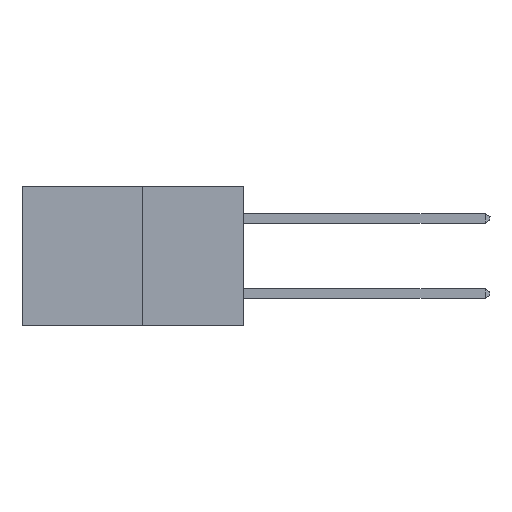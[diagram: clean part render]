
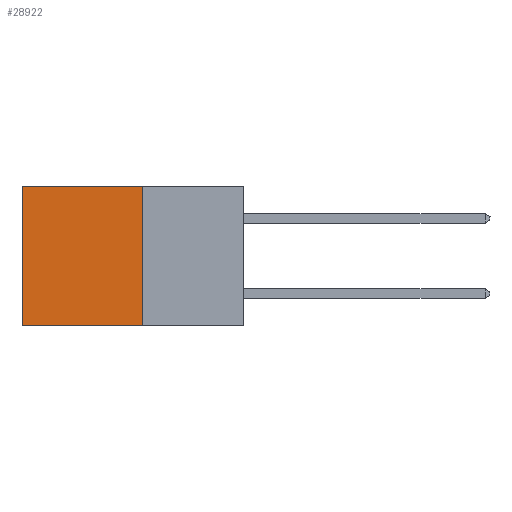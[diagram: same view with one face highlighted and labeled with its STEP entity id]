
A CAD part, left-side view. The second image highlights one B-rep face of the part: STEP entity #28922.
In plain terms, the highlighted planar face has unit normal (-1, 0, 0).
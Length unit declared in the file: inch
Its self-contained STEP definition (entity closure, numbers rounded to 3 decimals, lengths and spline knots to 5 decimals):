
#499 = CARTESIAN_POINT ( 'NONE',  ( 0.277, 0.59, 0. ) ) ;
#1030 = DIRECTION ( 'NONE',  ( 0., 0., -1. ) ) ;
#1636 = DIRECTION ( 'NONE',  ( 0., 0., -1. ) ) ;
#2954 = LINE ( 'NONE', #26502, #8799 ) ;
#3032 = LINE ( 'NONE', #10955, #22150 ) ;
#5028 = VECTOR ( 'NONE', #32125, 39.37008 ) ;
#6958 = PLANE ( 'NONE',  #21316 ) ;
#8799 = VECTOR ( 'NONE', #9034, 39.37008 ) ;
#9034 = DIRECTION ( 'NONE',  ( 0., 1., 0. ) ) ;
#10135 = ORIENTED_EDGE ( 'NONE', *, *, #14363, .F. ) ;
#10955 = CARTESIAN_POINT ( 'NONE',  ( 0.277, 0.27, -0.37 ) ) ;
#11963 = CARTESIAN_POINT ( 'NONE',  ( 0.277, 0.27, -0.37 ) ) ;
#12255 = ORIENTED_EDGE ( 'NONE', *, *, #31944, .T. ) ;
#13295 = FACE_OUTER_BOUND ( 'NONE', #19484, .T. ) ;
#14037 = EDGE_CURVE ( 'NONE', #16642, #22897, #18237, .T. ) ;
#14363 = EDGE_CURVE ( 'NONE', #31756, #16642, #3032, .T. ) ;
#14492 = DIRECTION ( 'NONE',  ( 0., 0., -1. ) ) ;
#15613 = VECTOR ( 'NONE', #1636, 39.37008 ) ;
#16126 = VERTEX_POINT ( 'NONE', #499 ) ;
#16642 = VERTEX_POINT ( 'NONE', #24701 ) ;
#17510 = ORIENTED_EDGE ( 'NONE', *, *, #14037, .F. ) ;
#18237 = LINE ( 'NONE', #29688, #5028 ) ;
#19066 = CARTESIAN_POINT ( 'NONE',  ( 0.277, 0.59, -0.37 ) ) ;
#19484 = EDGE_LOOP ( 'NONE', ( #27511, #17510, #10135, #12255 ) ) ;
#19878 = CARTESIAN_POINT ( 'NONE',  ( 0.277, 0.59, -0.37 ) ) ;
#21316 = AXIS2_PLACEMENT_3D ( 'NONE', #11963, #29379, #14492 ) ;
#21975 = EDGE_CURVE ( 'NONE', #16126, #22897, #28876, .T. ) ;
#22150 = VECTOR ( 'NONE', #1030, 39.37008 ) ;
#22897 = VERTEX_POINT ( 'NONE', #19878 ) ;
#24701 = CARTESIAN_POINT ( 'NONE',  ( 0.277, 0.27, -0.37 ) ) ;
#26502 = CARTESIAN_POINT ( 'NONE',  ( 0.277, 0.27, 0. ) ) ;
#27511 = ORIENTED_EDGE ( 'NONE', *, *, #21975, .T. ) ;
#28876 = LINE ( 'NONE', #19066, #15613 ) ;
#28922 = ADVANCED_FACE ( 'NONE', ( #13295 ), #6958, .F. ) ;
#29379 = DIRECTION ( 'NONE',  ( 1., 0., 0. ) ) ;
#29688 = CARTESIAN_POINT ( 'NONE',  ( 0.277, 0.27, -0.37 ) ) ;
#30771 = CARTESIAN_POINT ( 'NONE',  ( 0.277, 0.27, 0. ) ) ;
#31756 = VERTEX_POINT ( 'NONE', #30771 ) ;
#31944 = EDGE_CURVE ( 'NONE', #31756, #16126, #2954, .T. ) ;
#32125 = DIRECTION ( 'NONE',  ( 0., 1., 0. ) ) ;
